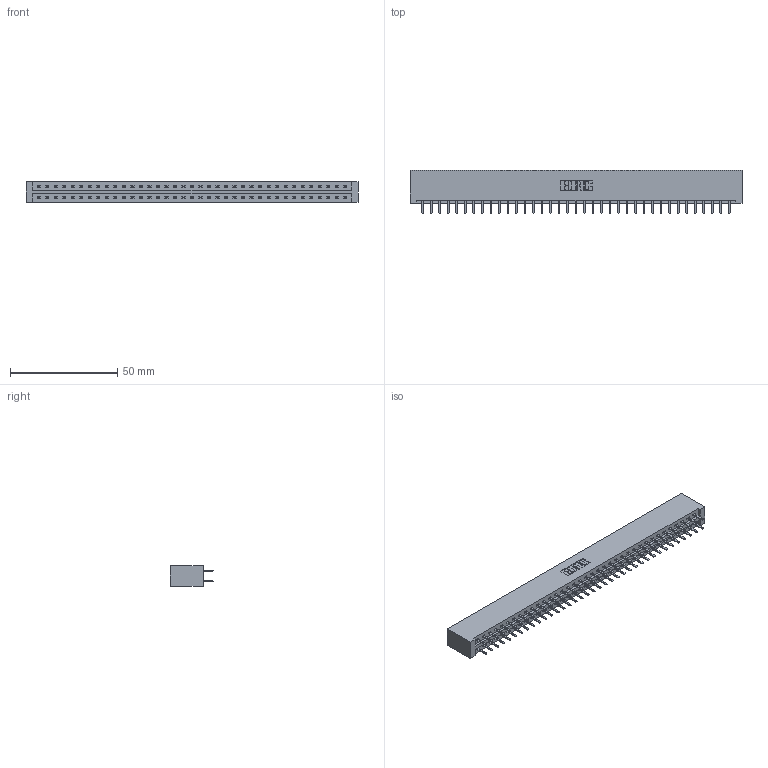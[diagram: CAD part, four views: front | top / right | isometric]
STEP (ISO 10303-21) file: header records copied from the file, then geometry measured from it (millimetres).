
FILE_DESCRIPTION (( 'STEP AP203' ), '1' );
FILE_NAME ('337-074-520-201.STEP', '2018-08-11T16:25:08', ( '' ), ( '' ), 'SwSTEP 2.0', 'SolidWorks 2016', '' );
FILE_SCHEMA (( 'CONFIG_CONTROL_DESIGN' ));
Length unit declared in the file: inch
Products named in the file (3): 337 Part_No Mounting Lugs; 345-292-001_345-293-120; 337-074-520-201
Assembly tree (75 placements, depth 2):
  337-074-520-201
    337 Part_No Mounting Lugs
    345-292-001_345-293-120  x74
Bounding box: 154.48 x 20.02 x 9.4 mm (x, y, z)
Volume: 16942.3 mm3; surface area: 19068 mm2
Topology: 75 solids, 75 shells, 4398 faces, 12793 edges, 8330 vertices
Faces by surface type: plane 3026, cylinder 1372
Entity records: 29171 total; most frequent: CARTESIAN_POINT 4930, ORIENTED_EDGE 4854, DIRECTION 4183, EDGE_CURVE 2427, LINE 2303, VECTOR 2303, VERTEX_POINT 1614, AXIS2_PLACEMENT_3D 940
